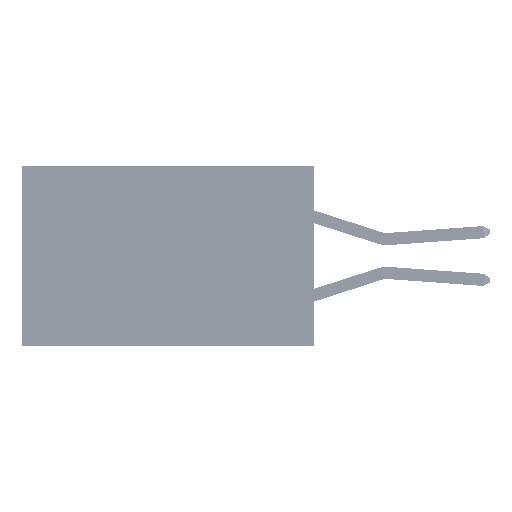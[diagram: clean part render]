
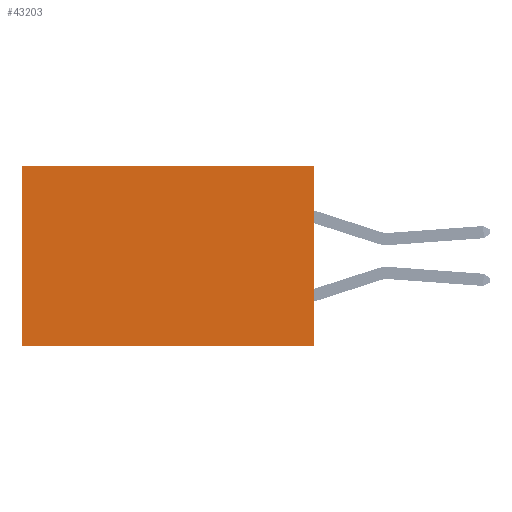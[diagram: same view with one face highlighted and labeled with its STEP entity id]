
A CAD part, left-side view. The second image highlights one B-rep face of the part: STEP entity #43203.
In plain terms, the highlighted planar face has unit normal (-1, 0, 0).
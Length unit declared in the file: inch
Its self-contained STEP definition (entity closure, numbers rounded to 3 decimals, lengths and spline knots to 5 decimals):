
#1305 = EDGE_CURVE ( 'NONE', #5741, #36864, #12137, .T. ) ;
#5741 = VERTEX_POINT ( 'NONE', #8493 ) ;
#8357 = ORIENTED_EDGE ( 'NONE', *, *, #28593, .T. ) ;
#8493 = CARTESIAN_POINT ( 'NONE',  ( 0.2875, 0., 0. ) ) ;
#8996 = CARTESIAN_POINT ( 'NONE',  ( 0.2875, 0., -0.37 ) ) ;
#10520 = ORIENTED_EDGE ( 'NONE', *, *, #1305, .T. ) ;
#12137 = LINE ( 'NONE', #12542, #44272 ) ;
#12542 = CARTESIAN_POINT ( 'NONE',  ( 0.2875, 0., 0. ) ) ;
#13450 = DIRECTION ( 'NONE',  ( 1., 0., 0. ) ) ;
#15526 = CARTESIAN_POINT ( 'NONE',  ( 0.2875, 0.6, 0. ) ) ;
#15793 = LINE ( 'NONE', #45689, #36246 ) ;
#16412 = DIRECTION ( 'NONE',  ( 0., 1., 0. ) ) ;
#16860 = ORIENTED_EDGE ( 'NONE', *, *, #35734, .F. ) ;
#17148 = DIRECTION ( 'NONE',  ( 0., 0., -1. ) ) ;
#18160 = LINE ( 'NONE', #15526, #37495 ) ;
#20055 = VERTEX_POINT ( 'NONE', #41414 ) ;
#20605 = PLANE ( 'NONE',  #41761 ) ;
#22082 = LINE ( 'NONE', #8996, #37538 ) ;
#24319 = CARTESIAN_POINT ( 'NONE',  ( 0.2875, 0., 0. ) ) ;
#24770 = DIRECTION ( 'NONE',  ( 0., 0., -1. ) ) ;
#26409 = DIRECTION ( 'NONE',  ( 0., 0., -1. ) ) ;
#27000 = CARTESIAN_POINT ( 'NONE',  ( 0.2875, 0.6, 0. ) ) ;
#27661 = CARTESIAN_POINT ( 'NONE',  ( 0.2875, 0., -0.37 ) ) ;
#28593 = EDGE_CURVE ( 'NONE', #36864, #20055, #18160, .T. ) ;
#28833 = ORIENTED_EDGE ( 'NONE', *, *, #32268, .F. ) ;
#29989 = FACE_OUTER_BOUND ( 'NONE', #43352, .T. ) ;
#32268 = EDGE_CURVE ( 'NONE', #5741, #39516, #15793, .T. ) ;
#33905 = DIRECTION ( 'NONE',  ( 0., 1., 0. ) ) ;
#35734 = EDGE_CURVE ( 'NONE', #39516, #20055, #22082, .T. ) ;
#36246 = VECTOR ( 'NONE', #24770, 39.37008 ) ;
#36864 = VERTEX_POINT ( 'NONE', #27000 ) ;
#37495 = VECTOR ( 'NONE', #26409, 39.37008 ) ;
#37538 = VECTOR ( 'NONE', #33905, 39.37008 ) ;
#39516 = VERTEX_POINT ( 'NONE', #27661 ) ;
#41414 = CARTESIAN_POINT ( 'NONE',  ( 0.2875, 0.6, -0.37 ) ) ;
#41761 = AXIS2_PLACEMENT_3D ( 'NONE', #24319, #13450, #17148 ) ;
#43203 = ADVANCED_FACE ( 'NONE', ( #29989 ), #20605, .F. ) ;
#43352 = EDGE_LOOP ( 'NONE', ( #8357, #16860, #28833, #10520 ) ) ;
#44272 = VECTOR ( 'NONE', #16412, 39.37008 ) ;
#45689 = CARTESIAN_POINT ( 'NONE',  ( 0.2875, 0., 0. ) ) ;
